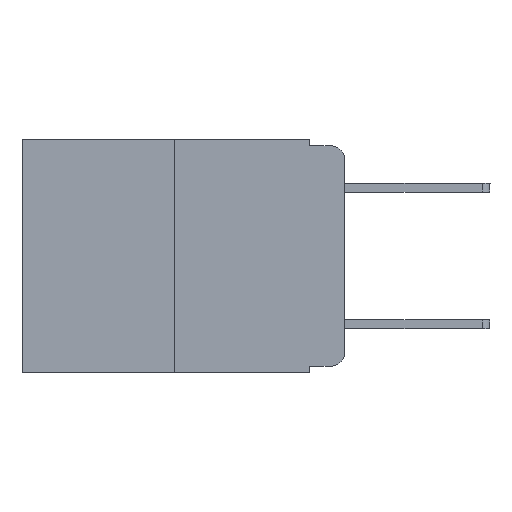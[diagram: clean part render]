
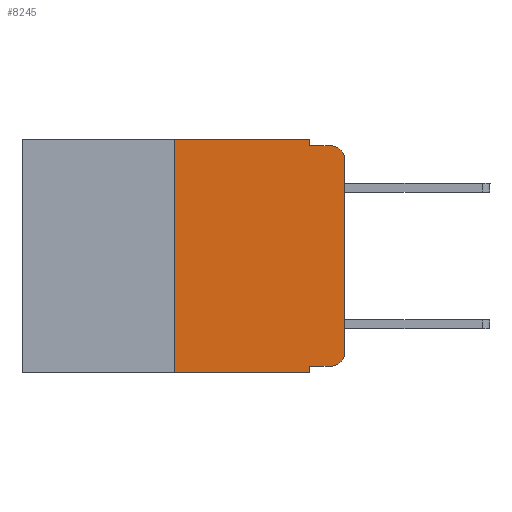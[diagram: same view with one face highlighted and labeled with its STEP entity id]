
A CAD part, left-side view. The second image highlights one B-rep face of the part: STEP entity #8245.
In plain terms, the highlighted planar face has unit normal (-1, 0, 0).
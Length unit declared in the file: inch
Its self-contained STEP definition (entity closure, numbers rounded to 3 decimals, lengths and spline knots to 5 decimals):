
#567 = CARTESIAN_POINT ( 'NONE',  ( 0., 0.051, 0. ) ) ;
#716 = CARTESIAN_POINT ( 'NONE',  ( 0., 0.02, -0.313 ) ) ;
#1055 = ORIENTED_EDGE ( 'NONE', *, *, #7839, .T. ) ;
#1137 = DIRECTION ( 'NONE',  ( 0., -1., 0. ) ) ;
#1225 = CARTESIAN_POINT ( 'NONE',  ( 0., 0.473, 0. ) ) ;
#1639 = AXIS2_PLACEMENT_3D ( 'NONE', #716, #20122, #18224 ) ;
#1778 = VECTOR ( 'NONE', #14524, 39.37008 ) ;
#2508 = DIRECTION ( 'NONE',  ( 0., 0., 1. ) ) ;
#2596 = VECTOR ( 'NONE', #8607, 39.37008 ) ;
#2622 = EDGE_CURVE ( 'NONE', #19348, #13328, #4966, .T. ) ;
#2977 = EDGE_CURVE ( 'NONE', #16031, #9471, #10522, .T. ) ;
#2992 = ORIENTED_EDGE ( 'NONE', *, *, #21254, .T. ) ;
#3982 = ORIENTED_EDGE ( 'NONE', *, *, #11563, .F. ) ;
#4245 = CARTESIAN_POINT ( 'NONE',  ( 0., 0.051, 0. ) ) ;
#4719 = ORIENTED_EDGE ( 'NONE', *, *, #24036, .F. ) ;
#4966 = LINE ( 'NONE', #12690, #21614 ) ;
#5091 = CARTESIAN_POINT ( 'NONE',  ( 0., 0.051, -0.343 ) ) ;
#5576 = VECTOR ( 'NONE', #18721, 39.37008 ) ;
#6115 = AXIS2_PLACEMENT_3D ( 'NONE', #14230, #21981, #20061 ) ;
#6509 = PLANE ( 'NONE',  #6115 ) ;
#6800 = CARTESIAN_POINT ( 'NONE',  ( 0., 0., 0. ) ) ;
#7045 = CARTESIAN_POINT ( 'NONE',  ( 0., 0.051, -0.333 ) ) ;
#7839 = EDGE_CURVE ( 'NONE', #9471, #19962, #20279, .T. ) ;
#7997 = CARTESIAN_POINT ( 'NONE',  ( 0., 0.25, 0. ) ) ;
#8050 = VECTOR ( 'NONE', #2508, 39.37008 ) ;
#8211 = ORIENTED_EDGE ( 'NONE', *, *, #2622, .F. ) ;
#8245 = ADVANCED_FACE ( 'NONE', ( #12208 ), #6509, .F. ) ;
#8307 = DIRECTION ( 'NONE',  ( 0., 0., -1. ) ) ;
#8605 = DIRECTION ( 'NONE',  ( 0., -1., 0. ) ) ;
#8607 = DIRECTION ( 'NONE',  ( 0., -1., 0. ) ) ;
#9314 = LINE ( 'NONE', #16907, #18658 ) ;
#9471 = VERTEX_POINT ( 'NONE', #9964 ) ;
#9791 = EDGE_CURVE ( 'NONE', #16031, #10368, #9314, .T. ) ;
#9934 = CIRCLE ( 'NONE', #17618, 0.02 ) ;
#9964 = CARTESIAN_POINT ( 'NONE',  ( 0., 0.02, -0.333 ) ) ;
#10368 = VERTEX_POINT ( 'NONE', #5091 ) ;
#10410 = DIRECTION ( 'NONE',  ( 0., 0., -1. ) ) ;
#10514 = CARTESIAN_POINT ( 'NONE',  ( 0., 0.051, -0.01 ) ) ;
#10522 = LINE ( 'NONE', #14561, #17264 ) ;
#10589 = EDGE_CURVE ( 'NONE', #18163, #13328, #9934, .T. ) ;
#10637 = LINE ( 'NONE', #1225, #5576 ) ;
#11557 = CARTESIAN_POINT ( 'NONE',  ( 0., 0., -0.313 ) ) ;
#11563 = EDGE_CURVE ( 'NONE', #21531, #19348, #17946, .T. ) ;
#12208 = FACE_OUTER_BOUND ( 'NONE', #14028, .T. ) ;
#12560 = CARTESIAN_POINT ( 'NONE',  ( 0., 0.02, -0.03 ) ) ;
#12690 = CARTESIAN_POINT ( 'NONE',  ( 0., 0.051, -0.01 ) ) ;
#13328 = VERTEX_POINT ( 'NONE', #24517 ) ;
#13666 = ORIENTED_EDGE ( 'NONE', *, *, #10589, .T. ) ;
#13792 = ORIENTED_EDGE ( 'NONE', *, *, #13804, .F. ) ;
#13804 = EDGE_CURVE ( 'NONE', #13899, #23384, #21786, .T. ) ;
#13899 = VERTEX_POINT ( 'NONE', #23829 ) ;
#14028 = EDGE_LOOP ( 'NONE', ( #2992, #13666, #8211, #3982, #4719, #13792, #20139, #20035, #24860, #1055 ) ) ;
#14230 = CARTESIAN_POINT ( 'NONE',  ( 0., 0.473, 0. ) ) ;
#14524 = DIRECTION ( 'NONE',  ( 0., 0., 1. ) ) ;
#14561 = CARTESIAN_POINT ( 'NONE',  ( 0., 0.051, -0.333 ) ) ;
#14563 = LINE ( 'NONE', #16704, #2596 ) ;
#16031 = VERTEX_POINT ( 'NONE', #7045 ) ;
#16704 = CARTESIAN_POINT ( 'NONE',  ( 0., 0.473, -0.343 ) ) ;
#16907 = CARTESIAN_POINT ( 'NONE',  ( 0., 0.051, 0. ) ) ;
#17264 = VECTOR ( 'NONE', #8605, 39.37008 ) ;
#17618 = AXIS2_PLACEMENT_3D ( 'NONE', #12560, #21959, #10410 ) ;
#17946 = LINE ( 'NONE', #567, #24160 ) ;
#17974 = CARTESIAN_POINT ( 'NONE',  ( 0., 0.25, 0. ) ) ;
#18163 = VERTEX_POINT ( 'NONE', #25048 ) ;
#18224 = DIRECTION ( 'NONE',  ( 0., 0., -1. ) ) ;
#18658 = VECTOR ( 'NONE', #20967, 39.37008 ) ;
#18721 = DIRECTION ( 'NONE',  ( 0., -1., 0. ) ) ;
#19348 = VERTEX_POINT ( 'NONE', #10514 ) ;
#19962 = VERTEX_POINT ( 'NONE', #11557 ) ;
#20035 = ORIENTED_EDGE ( 'NONE', *, *, #9791, .F. ) ;
#20061 = DIRECTION ( 'NONE',  ( 0., 0., -1. ) ) ;
#20122 = DIRECTION ( 'NONE',  ( -1., 0., 0. ) ) ;
#20139 = ORIENTED_EDGE ( 'NONE', *, *, #22033, .T. ) ;
#20279 = CIRCLE ( 'NONE', #1639, 0.02 ) ;
#20967 = DIRECTION ( 'NONE',  ( 0., 0., -1. ) ) ;
#21254 = EDGE_CURVE ( 'NONE', #19962, #18163, #24188, .T. ) ;
#21531 = VERTEX_POINT ( 'NONE', #4245 ) ;
#21614 = VECTOR ( 'NONE', #1137, 39.37008 ) ;
#21786 = LINE ( 'NONE', #17974, #8050 ) ;
#21959 = DIRECTION ( 'NONE',  ( -1., 0., 0. ) ) ;
#21981 = DIRECTION ( 'NONE',  ( 1., 0., 0. ) ) ;
#22033 = EDGE_CURVE ( 'NONE', #13899, #10368, #14563, .T. ) ;
#23384 = VERTEX_POINT ( 'NONE', #7997 ) ;
#23829 = CARTESIAN_POINT ( 'NONE',  ( 0., 0.25, -0.343 ) ) ;
#24036 = EDGE_CURVE ( 'NONE', #23384, #21531, #10637, .T. ) ;
#24160 = VECTOR ( 'NONE', #8307, 39.37008 ) ;
#24188 = LINE ( 'NONE', #6800, #1778 ) ;
#24517 = CARTESIAN_POINT ( 'NONE',  ( 0., 0.02, -0.01 ) ) ;
#24860 = ORIENTED_EDGE ( 'NONE', *, *, #2977, .T. ) ;
#25048 = CARTESIAN_POINT ( 'NONE',  ( 0., 0., -0.03 ) ) ;
